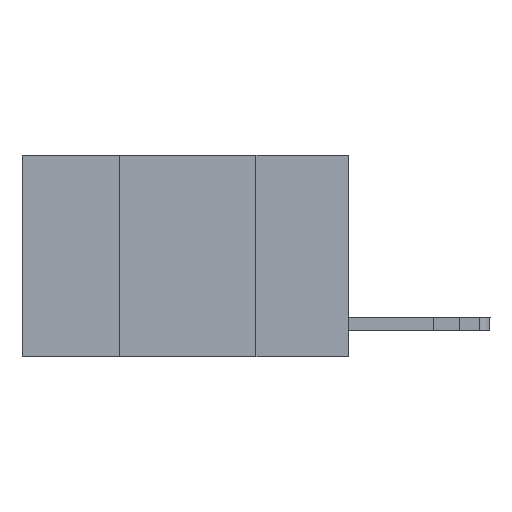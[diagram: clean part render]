
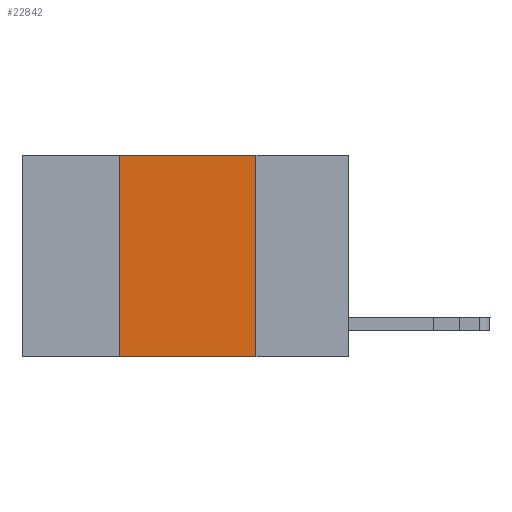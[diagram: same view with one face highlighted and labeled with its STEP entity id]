
A CAD part, left-side view. The second image highlights one B-rep face of the part: STEP entity #22842.
In plain terms, the highlighted planar face has unit normal (-1, 0, 0).
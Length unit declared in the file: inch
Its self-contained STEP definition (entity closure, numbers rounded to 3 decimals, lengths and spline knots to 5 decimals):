
#505 = LINE ( 'NONE', #6003, #16960 ) ;
#624 = VERTEX_POINT ( 'NONE', #24318 ) ;
#629 = VECTOR ( 'NONE', #17125, 39.37008 ) ;
#950 = VERTEX_POINT ( 'NONE', #8186 ) ;
#1948 = CARTESIAN_POINT ( 'NONE',  ( 0., 0.17, 0. ) ) ;
#2623 = VECTOR ( 'NONE', #8345, 39.37008 ) ;
#3684 = DIRECTION ( 'NONE',  ( 0., -1., 0. ) ) ;
#3775 = VERTEX_POINT ( 'NONE', #9167 ) ;
#5154 = ORIENTED_EDGE ( 'NONE', *, *, #21454, .F. ) ;
#6003 = CARTESIAN_POINT ( 'NONE',  ( 0., 0.6, 0. ) ) ;
#6308 = DIRECTION ( 'NONE',  ( 0., 0., -1. ) ) ;
#8186 = CARTESIAN_POINT ( 'NONE',  ( 0., 0.42, 0. ) ) ;
#8345 = DIRECTION ( 'NONE',  ( 0., 0., -1. ) ) ;
#8732 = EDGE_CURVE ( 'NONE', #624, #3775, #20439, .T. ) ;
#9167 = CARTESIAN_POINT ( 'NONE',  ( 0., 0.17, -0.37 ) ) ;
#9799 = VECTOR ( 'NONE', #3684, 39.37008 ) ;
#12067 = LINE ( 'NONE', #25802, #629 ) ;
#12872 = ORIENTED_EDGE ( 'NONE', *, *, #15896, .F. ) ;
#13901 = AXIS2_PLACEMENT_3D ( 'NONE', #16979, #19144, #6308 ) ;
#14453 = EDGE_CURVE ( 'NONE', #26503, #3775, #21189, .T. ) ;
#14816 = PLANE ( 'NONE',  #13901 ) ;
#15187 = ORIENTED_EDGE ( 'NONE', *, *, #8732, .F. ) ;
#15896 = EDGE_CURVE ( 'NONE', #26503, #950, #12067, .T. ) ;
#16603 = FACE_OUTER_BOUND ( 'NONE', #17754, .T. ) ;
#16960 = VECTOR ( 'NONE', #20985, 39.37008 ) ;
#16979 = CARTESIAN_POINT ( 'NONE',  ( 0., 0.6, 0. ) ) ;
#17125 = DIRECTION ( 'NONE',  ( 0., 0., 1. ) ) ;
#17754 = EDGE_LOOP ( 'NONE', ( #15187, #5154, #12872, #24964 ) ) ;
#18518 = CARTESIAN_POINT ( 'NONE',  ( 0., 0.42, -0.37 ) ) ;
#19144 = DIRECTION ( 'NONE',  ( 1., 0., 0. ) ) ;
#20439 = LINE ( 'NONE', #1948, #2623 ) ;
#20985 = DIRECTION ( 'NONE',  ( 0., -1., 0. ) ) ;
#21189 = LINE ( 'NONE', #23019, #9799 ) ;
#21454 = EDGE_CURVE ( 'NONE', #950, #624, #505, .T. ) ;
#22842 = ADVANCED_FACE ( 'NONE', ( #16603 ), #14816, .F. ) ;
#23019 = CARTESIAN_POINT ( 'NONE',  ( 0., 0.6, -0.37 ) ) ;
#24318 = CARTESIAN_POINT ( 'NONE',  ( 0., 0.17, 0. ) ) ;
#24964 = ORIENTED_EDGE ( 'NONE', *, *, #14453, .T. ) ;
#25802 = CARTESIAN_POINT ( 'NONE',  ( 0., 0.42, 0. ) ) ;
#26503 = VERTEX_POINT ( 'NONE', #18518 ) ;
